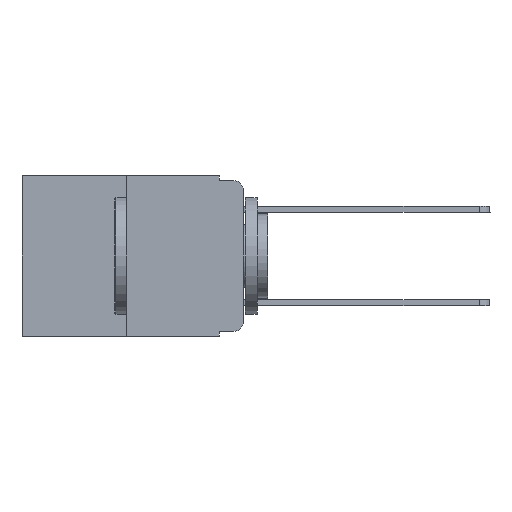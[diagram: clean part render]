
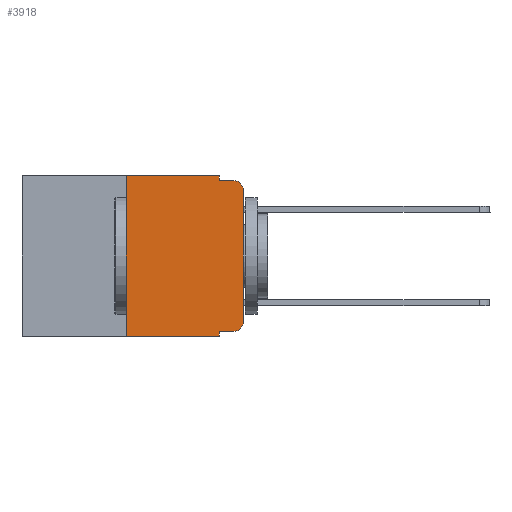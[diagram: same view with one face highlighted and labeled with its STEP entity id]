
A CAD part, left-side view. The second image highlights one B-rep face of the part: STEP entity #3918.
In plain terms, the highlighted planar face has unit normal (-1, 0, 0).
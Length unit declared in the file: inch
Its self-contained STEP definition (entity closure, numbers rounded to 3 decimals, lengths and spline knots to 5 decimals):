
#48 = VECTOR ( 'NONE', #9956, 39.37008 ) ;
#163 = ORIENTED_EDGE ( 'NONE', *, *, #10532, .T. ) ;
#454 = CIRCLE ( 'NONE', #1979, 0.02 ) ;
#832 = CARTESIAN_POINT ( 'NONE',  ( 0., 0.25, 0. ) ) ;
#978 = LINE ( 'NONE', #5400, #9620 ) ;
#1316 = DIRECTION ( 'NONE',  ( 0., 0., 1. ) ) ;
#1539 = LINE ( 'NONE', #8145, #9905 ) ;
#1670 = ORIENTED_EDGE ( 'NONE', *, *, #10791, .T. ) ;
#1722 = CARTESIAN_POINT ( 'NONE',  ( 0., 0., -0.03 ) ) ;
#1917 = DIRECTION ( 'NONE',  ( 0., 0., -1. ) ) ;
#1979 = AXIS2_PLACEMENT_3D ( 'NONE', #2611, #3411, #8477 ) ;
#2013 = LINE ( 'NONE', #9226, #10648 ) ;
#2074 = CARTESIAN_POINT ( 'NONE',  ( 0., 0.051, -0.333 ) ) ;
#2121 = LINE ( 'NONE', #2940, #6591 ) ;
#2150 = CARTESIAN_POINT ( 'NONE',  ( 0., 0.473, 0. ) ) ;
#2158 = EDGE_CURVE ( 'NONE', #7335, #4638, #8459, .T. ) ;
#2261 = LINE ( 'NONE', #6763, #8675 ) ;
#2464 = VERTEX_POINT ( 'NONE', #1722 ) ;
#2477 = ORIENTED_EDGE ( 'NONE', *, *, #3789, .F. ) ;
#2532 = CARTESIAN_POINT ( 'NONE',  ( 0., 0.02, -0.01 ) ) ;
#2611 = CARTESIAN_POINT ( 'NONE',  ( 0., 0.02, -0.03 ) ) ;
#2735 = VERTEX_POINT ( 'NONE', #3562 ) ;
#2833 = DIRECTION ( 'NONE',  ( 0., 0., -1. ) ) ;
#2940 = CARTESIAN_POINT ( 'NONE',  ( 0., 0.051, 0. ) ) ;
#3196 = VERTEX_POINT ( 'NONE', #9465 ) ;
#3411 = DIRECTION ( 'NONE',  ( -1., 0., 0. ) ) ;
#3562 = CARTESIAN_POINT ( 'NONE',  ( 0., 0.051, -0.343 ) ) ;
#3789 = EDGE_CURVE ( 'NONE', #3196, #5210, #6717, .T. ) ;
#3918 = ADVANCED_FACE ( 'NONE', ( #8670 ), #4084, .F. ) ;
#4084 = PLANE ( 'NONE',  #4472 ) ;
#4199 = CARTESIAN_POINT ( 'NONE',  ( 0., 0.02, -0.333 ) ) ;
#4412 = VERTEX_POINT ( 'NONE', #832 ) ;
#4472 = AXIS2_PLACEMENT_3D ( 'NONE', #2150, #7744, #1917 ) ;
#4557 = DIRECTION ( 'NONE',  ( 0., -1., 0. ) ) ;
#4634 = CARTESIAN_POINT ( 'NONE',  ( 0., 0.02, -0.313 ) ) ;
#4638 = VERTEX_POINT ( 'NONE', #5233 ) ;
#4696 = CARTESIAN_POINT ( 'NONE',  ( 0., 0.051, 0. ) ) ;
#4759 = CARTESIAN_POINT ( 'NONE',  ( 0., 0., 0. ) ) ;
#4847 = DIRECTION ( 'NONE',  ( 0., -1., 0. ) ) ;
#5040 = ORIENTED_EDGE ( 'NONE', *, *, #5728, .F. ) ;
#5041 = EDGE_LOOP ( 'NONE', ( #163, #1670, #2477, #7376, #5040, #7743, #6123, #10613, #9413, #10569 ) ) ;
#5210 = VERTEX_POINT ( 'NONE', #2532 ) ;
#5233 = CARTESIAN_POINT ( 'NONE',  ( 0., 0., -0.313 ) ) ;
#5400 = CARTESIAN_POINT ( 'NONE',  ( 0., 0.473, 0. ) ) ;
#5411 = DIRECTION ( 'NONE',  ( -1., 0., 0. ) ) ;
#5728 = EDGE_CURVE ( 'NONE', #4412, #10533, #978, .T. ) ;
#6123 = ORIENTED_EDGE ( 'NONE', *, *, #10293, .T. ) ;
#6329 = VECTOR ( 'NONE', #4847, 39.37008 ) ;
#6389 = DIRECTION ( 'NONE',  ( 0., 0., -1. ) ) ;
#6441 = EDGE_CURVE ( 'NONE', #10533, #3196, #2121, .T. ) ;
#6591 = VECTOR ( 'NONE', #2833, 39.37008 ) ;
#6603 = LINE ( 'NONE', #10666, #6329 ) ;
#6717 = LINE ( 'NONE', #9097, #48 ) ;
#6763 = CARTESIAN_POINT ( 'NONE',  ( 0., 0.25, 0. ) ) ;
#7026 = VERTEX_POINT ( 'NONE', #2074 ) ;
#7204 = CARTESIAN_POINT ( 'NONE',  ( 0., 0.25, -0.343 ) ) ;
#7250 = VECTOR ( 'NONE', #1316, 39.37008 ) ;
#7335 = VERTEX_POINT ( 'NONE', #4199 ) ;
#7342 = EDGE_CURVE ( 'NONE', #9929, #4412, #2261, .T. ) ;
#7376 = ORIENTED_EDGE ( 'NONE', *, *, #6441, .F. ) ;
#7743 = ORIENTED_EDGE ( 'NONE', *, *, #7342, .F. ) ;
#7744 = DIRECTION ( 'NONE',  ( 1., 0., 0. ) ) ;
#8145 = CARTESIAN_POINT ( 'NONE',  ( 0., 0.051, 0. ) ) ;
#8459 = CIRCLE ( 'NONE', #10645, 0.02 ) ;
#8477 = DIRECTION ( 'NONE',  ( 0., 0., -1. ) ) ;
#8670 = FACE_OUTER_BOUND ( 'NONE', #5041, .T. ) ;
#8675 = VECTOR ( 'NONE', #10150, 39.37008 ) ;
#8810 = EDGE_CURVE ( 'NONE', #7026, #2735, #1539, .T. ) ;
#9097 = CARTESIAN_POINT ( 'NONE',  ( 0., 0.051, -0.01 ) ) ;
#9226 = CARTESIAN_POINT ( 'NONE',  ( 0., 0.473, -0.343 ) ) ;
#9413 = ORIENTED_EDGE ( 'NONE', *, *, #10057, .T. ) ;
#9465 = CARTESIAN_POINT ( 'NONE',  ( 0., 0.051, -0.01 ) ) ;
#9620 = VECTOR ( 'NONE', #4557, 39.37008 ) ;
#9905 = VECTOR ( 'NONE', #6389, 39.37008 ) ;
#9929 = VERTEX_POINT ( 'NONE', #7204 ) ;
#9956 = DIRECTION ( 'NONE',  ( 0., -1., 0. ) ) ;
#9968 = DIRECTION ( 'NONE',  ( 0., -1., 0. ) ) ;
#10057 = EDGE_CURVE ( 'NONE', #7026, #7335, #6603, .T. ) ;
#10150 = DIRECTION ( 'NONE',  ( 0., 0., 1. ) ) ;
#10260 = LINE ( 'NONE', #4759, #7250 ) ;
#10293 = EDGE_CURVE ( 'NONE', #9929, #2735, #2013, .T. ) ;
#10491 = DIRECTION ( 'NONE',  ( 0., 0., -1. ) ) ;
#10532 = EDGE_CURVE ( 'NONE', #4638, #2464, #10260, .T. ) ;
#10533 = VERTEX_POINT ( 'NONE', #4696 ) ;
#10569 = ORIENTED_EDGE ( 'NONE', *, *, #2158, .T. ) ;
#10613 = ORIENTED_EDGE ( 'NONE', *, *, #8810, .F. ) ;
#10645 = AXIS2_PLACEMENT_3D ( 'NONE', #4634, #5411, #10491 ) ;
#10648 = VECTOR ( 'NONE', #9968, 39.37008 ) ;
#10666 = CARTESIAN_POINT ( 'NONE',  ( 0., 0.051, -0.333 ) ) ;
#10791 = EDGE_CURVE ( 'NONE', #2464, #5210, #454, .T. ) ;
